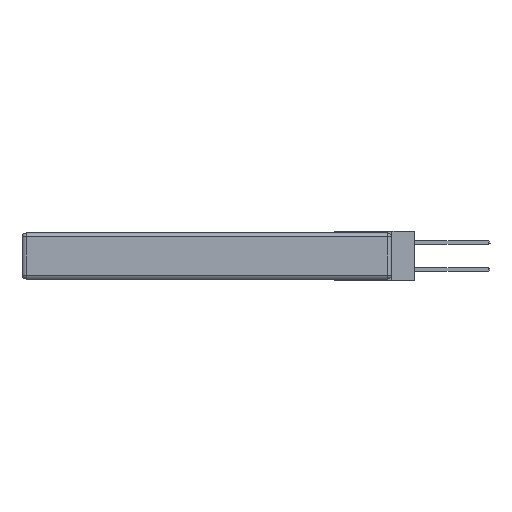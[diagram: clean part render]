
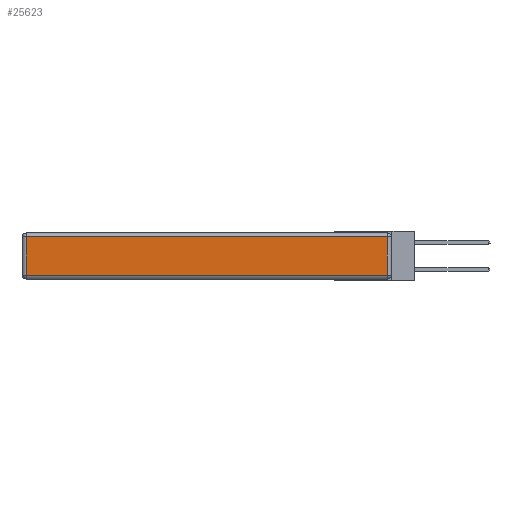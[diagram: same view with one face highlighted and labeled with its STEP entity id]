
A CAD part, left-side view. The second image highlights one B-rep face of the part: STEP entity #25623.
In plain terms, the highlighted planar face has unit normal (-1, 0, 0).
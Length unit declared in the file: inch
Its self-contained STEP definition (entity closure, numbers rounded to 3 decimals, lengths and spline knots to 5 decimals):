
#798 = PLANE ( 'NONE',  #8081 ) ;
#1817 = EDGE_LOOP ( 'NONE', ( #15358, #27982, #12857, #23695 ) ) ;
#3887 = LINE ( 'NONE', #28444, #4292 ) ;
#4292 = VECTOR ( 'NONE', #12976, 39.37008 ) ;
#5711 = FACE_OUTER_BOUND ( 'NONE', #1817, .T. ) ;
#5773 = LINE ( 'NONE', #23807, #25601 ) ;
#6593 = EDGE_CURVE ( 'NONE', #32539, #9650, #21137, .T. ) ;
#7363 = EDGE_CURVE ( 'NONE', #9650, #20361, #5773, .T. ) ;
#8081 = AXIS2_PLACEMENT_3D ( 'NONE', #8634, #8969, #14409 ) ;
#8215 = VECTOR ( 'NONE', #19611, 39.37008 ) ;
#8634 = CARTESIAN_POINT ( 'NONE',  ( 0., 0., -0.343 ) ) ;
#8969 = DIRECTION ( 'NONE',  ( -1., 0., 0. ) ) ;
#9650 = VERTEX_POINT ( 'NONE', #22284 ) ;
#12857 = ORIENTED_EDGE ( 'NONE', *, *, #7363, .T. ) ;
#12976 = DIRECTION ( 'NONE',  ( 0., 0., -1. ) ) ;
#13229 = CARTESIAN_POINT ( 'NONE',  ( 0., 2.72, -0.313 ) ) ;
#14409 = DIRECTION ( 'NONE',  ( 0., 0., 1. ) ) ;
#15358 = ORIENTED_EDGE ( 'NONE', *, *, #26562, .T. ) ;
#17963 = VERTEX_POINT ( 'NONE', #13229 ) ;
#19611 = DIRECTION ( 'NONE',  ( 0., 0., 1. ) ) ;
#20347 = CARTESIAN_POINT ( 'NONE',  ( 0., 0.03, -0.313 ) ) ;
#20361 = VERTEX_POINT ( 'NONE', #28782 ) ;
#21137 = LINE ( 'NONE', #32695, #8215 ) ;
#22284 = CARTESIAN_POINT ( 'NONE',  ( 0., 0.03, -0.03 ) ) ;
#23130 = CARTESIAN_POINT ( 'NONE',  ( 0., 0., -0.313 ) ) ;
#23695 = ORIENTED_EDGE ( 'NONE', *, *, #27272, .T. ) ;
#23807 = CARTESIAN_POINT ( 'NONE',  ( 0., 2.75, -0.03 ) ) ;
#25430 = LINE ( 'NONE', #23130, #28284 ) ;
#25601 = VECTOR ( 'NONE', #26427, 39.37008 ) ;
#25623 = ADVANCED_FACE ( 'NONE', ( #5711 ), #798, .T. ) ;
#26427 = DIRECTION ( 'NONE',  ( 0., 1., 0. ) ) ;
#26562 = EDGE_CURVE ( 'NONE', #17963, #32539, #25430, .T. ) ;
#27272 = EDGE_CURVE ( 'NONE', #20361, #17963, #3887, .T. ) ;
#27982 = ORIENTED_EDGE ( 'NONE', *, *, #6593, .T. ) ;
#28284 = VECTOR ( 'NONE', #28368, 39.37008 ) ;
#28368 = DIRECTION ( 'NONE',  ( 0., -1., 0. ) ) ;
#28444 = CARTESIAN_POINT ( 'NONE',  ( 0., 2.72, -0.343 ) ) ;
#28782 = CARTESIAN_POINT ( 'NONE',  ( 0., 2.72, -0.03 ) ) ;
#32539 = VERTEX_POINT ( 'NONE', #20347 ) ;
#32695 = CARTESIAN_POINT ( 'NONE',  ( 0., 0.03, -0.343 ) ) ;
